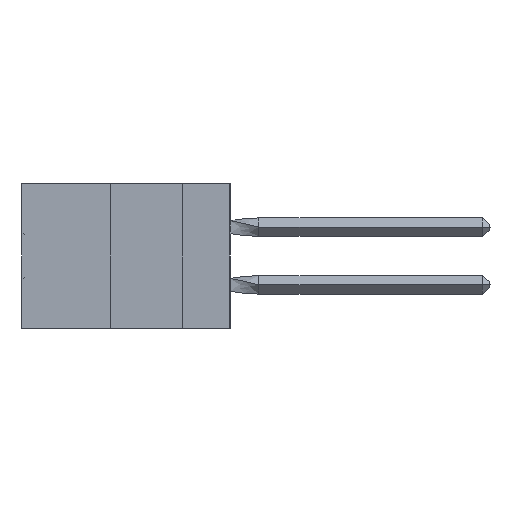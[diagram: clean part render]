
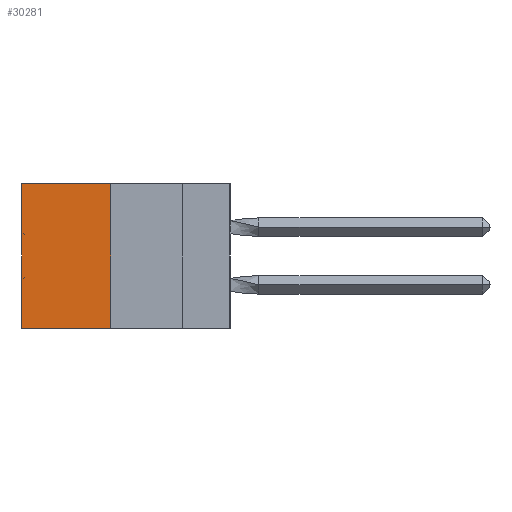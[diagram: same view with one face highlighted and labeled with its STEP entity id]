
A CAD part, left-side view. The second image highlights one B-rep face of the part: STEP entity #30281.
In plain terms, the highlighted planar face has unit normal (-1, 0, 0).
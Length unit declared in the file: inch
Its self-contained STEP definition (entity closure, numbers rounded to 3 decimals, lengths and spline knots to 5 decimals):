
#273 = VERTEX_POINT ( 'NONE', #48421 ) ;
#1862 = DIRECTION ( 'NONE',  ( 0., 0., -1. ) ) ;
#9300 = DIRECTION ( 'NONE',  ( 1., 0., 0. ) ) ;
#10356 = EDGE_LOOP ( 'NONE', ( #24271, #31557, #38682, #18259 ) ) ;
#11460 = DIRECTION ( 'NONE',  ( 0., 1., 0. ) ) ;
#13618 = VERTEX_POINT ( 'NONE', #26306 ) ;
#14584 = VECTOR ( 'NONE', #43354, 39.37008 ) ;
#15839 = VECTOR ( 'NONE', #16445, 39.37008 ) ;
#16445 = DIRECTION ( 'NONE',  ( 0., 1., 0. ) ) ;
#17074 = EDGE_CURVE ( 'NONE', #46443, #13618, #23390, .T. ) ;
#18165 = AXIS2_PLACEMENT_3D ( 'NONE', #47760, #9300, #21810 ) ;
#18259 = ORIENTED_EDGE ( 'NONE', *, *, #41582, .T. ) ;
#19852 = EDGE_CURVE ( 'NONE', #21232, #273, #34598, .T. ) ;
#20171 = CARTESIAN_POINT ( 'NONE',  ( 0.305, 0.413, -0.5 ) ) ;
#20730 = FACE_OUTER_BOUND ( 'NONE', #10356, .T. ) ;
#21232 = VERTEX_POINT ( 'NONE', #31202 ) ;
#21810 = DIRECTION ( 'NONE',  ( 0., 0., -1. ) ) ;
#23071 = LINE ( 'NONE', #46200, #49165 ) ;
#23390 = LINE ( 'NONE', #28849, #26474 ) ;
#24271 = ORIENTED_EDGE ( 'NONE', *, *, #17074, .T. ) ;
#26306 = CARTESIAN_POINT ( 'NONE',  ( 0.305, 0.72, -0.5 ) ) ;
#26474 = VECTOR ( 'NONE', #1862, 39.37008 ) ;
#27112 = CARTESIAN_POINT ( 'NONE',  ( 0.305, 0.72, 0. ) ) ;
#28849 = CARTESIAN_POINT ( 'NONE',  ( 0.305, 0.72, -0.5 ) ) ;
#30248 = EDGE_CURVE ( 'NONE', #273, #13618, #31031, .T. ) ;
#30281 = ADVANCED_FACE ( 'NONE', ( #20730 ), #36056, .F. ) ;
#31031 = LINE ( 'NONE', #20171, #15839 ) ;
#31202 = CARTESIAN_POINT ( 'NONE',  ( 0.305, 0.413, 0. ) ) ;
#31557 = ORIENTED_EDGE ( 'NONE', *, *, #30248, .F. ) ;
#34598 = LINE ( 'NONE', #47102, #14584 ) ;
#36056 = PLANE ( 'NONE',  #18165 ) ;
#38682 = ORIENTED_EDGE ( 'NONE', *, *, #19852, .F. ) ;
#41582 = EDGE_CURVE ( 'NONE', #21232, #46443, #23071, .T. ) ;
#43354 = DIRECTION ( 'NONE',  ( 0., 0., -1. ) ) ;
#46200 = CARTESIAN_POINT ( 'NONE',  ( 0.305, 0.413, 0. ) ) ;
#46443 = VERTEX_POINT ( 'NONE', #27112 ) ;
#47102 = CARTESIAN_POINT ( 'NONE',  ( 0.305, 0.413, -0.5 ) ) ;
#47760 = CARTESIAN_POINT ( 'NONE',  ( 0.305, 0.413, -0.5 ) ) ;
#48421 = CARTESIAN_POINT ( 'NONE',  ( 0.305, 0.413, -0.5 ) ) ;
#49165 = VECTOR ( 'NONE', #11460, 39.37008 ) ;
